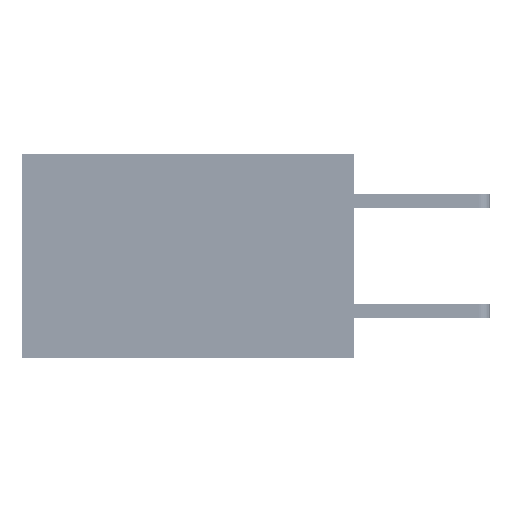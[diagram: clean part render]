
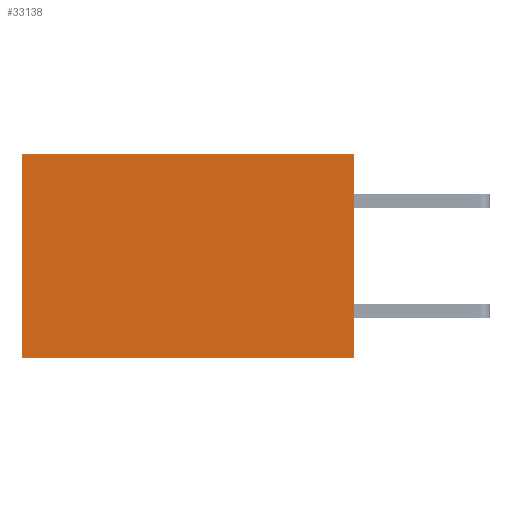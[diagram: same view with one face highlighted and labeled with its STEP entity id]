
A CAD part, left-side view. The second image highlights one B-rep face of the part: STEP entity #33138.
In plain terms, the highlighted planar face has unit normal (-1, 0, 0).
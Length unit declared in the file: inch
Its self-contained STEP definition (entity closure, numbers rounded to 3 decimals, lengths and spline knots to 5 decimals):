
#513 = VERTEX_POINT ( 'NONE', #34645 ) ;
#2575 = VECTOR ( 'NONE', #37362, 39.37008 ) ;
#3244 = CARTESIAN_POINT ( 'NONE',  ( 0.2875, 0.6, 0. ) ) ;
#3371 = PLANE ( 'NONE',  #43173 ) ;
#4369 = EDGE_CURVE ( 'NONE', #20301, #28312, #12614, .T. ) ;
#4533 = CARTESIAN_POINT ( 'NONE',  ( 0.2875, 0., -0.37 ) ) ;
#5950 = ORIENTED_EDGE ( 'NONE', *, *, #4369, .T. ) ;
#6014 = ORIENTED_EDGE ( 'NONE', *, *, #14369, .F. ) ;
#12614 = LINE ( 'NONE', #37134, #28929 ) ;
#14369 = EDGE_CURVE ( 'NONE', #513, #28312, #21870, .T. ) ;
#14379 = FACE_OUTER_BOUND ( 'NONE', #48932, .T. ) ;
#15227 = EDGE_CURVE ( 'NONE', #24507, #513, #36860, .T. ) ;
#15717 = DIRECTION ( 'NONE',  ( 1., 0., 0. ) ) ;
#18228 = VECTOR ( 'NONE', #35504, 39.37008 ) ;
#19206 = DIRECTION ( 'NONE',  ( 0., 0., -1. ) ) ;
#20129 = CARTESIAN_POINT ( 'NONE',  ( 0.2875, 0., 0. ) ) ;
#20301 = VERTEX_POINT ( 'NONE', #3244 ) ;
#21870 = LINE ( 'NONE', #4533, #18228 ) ;
#24507 = VERTEX_POINT ( 'NONE', #20129 ) ;
#28312 = VERTEX_POINT ( 'NONE', #31471 ) ;
#28391 = DIRECTION ( 'NONE',  ( 0., 0., -1. ) ) ;
#28929 = VECTOR ( 'NONE', #19206, 39.37008 ) ;
#29491 = ORIENTED_EDGE ( 'NONE', *, *, #15227, .F. ) ;
#30392 = LINE ( 'NONE', #48755, #2575 ) ;
#30405 = EDGE_CURVE ( 'NONE', #24507, #20301, #30392, .T. ) ;
#30598 = CARTESIAN_POINT ( 'NONE',  ( 0.2875, 0., 0. ) ) ;
#31102 = DIRECTION ( 'NONE',  ( 0., 0., -1. ) ) ;
#31471 = CARTESIAN_POINT ( 'NONE',  ( 0.2875, 0.6, -0.37 ) ) ;
#32511 = CARTESIAN_POINT ( 'NONE',  ( 0.2875, 0., 0. ) ) ;
#33138 = ADVANCED_FACE ( 'NONE', ( #14379 ), #3371, .F. ) ;
#33838 = ORIENTED_EDGE ( 'NONE', *, *, #30405, .T. ) ;
#34645 = CARTESIAN_POINT ( 'NONE',  ( 0.2875, 0., -0.37 ) ) ;
#35504 = DIRECTION ( 'NONE',  ( 0., 1., 0. ) ) ;
#36860 = LINE ( 'NONE', #32511, #42962 ) ;
#37134 = CARTESIAN_POINT ( 'NONE',  ( 0.2875, 0.6, 0. ) ) ;
#37362 = DIRECTION ( 'NONE',  ( 0., 1., 0. ) ) ;
#42962 = VECTOR ( 'NONE', #28391, 39.37008 ) ;
#43173 = AXIS2_PLACEMENT_3D ( 'NONE', #30598, #15717, #31102 ) ;
#48755 = CARTESIAN_POINT ( 'NONE',  ( 0.2875, 0., 0. ) ) ;
#48932 = EDGE_LOOP ( 'NONE', ( #5950, #6014, #29491, #33838 ) ) ;
